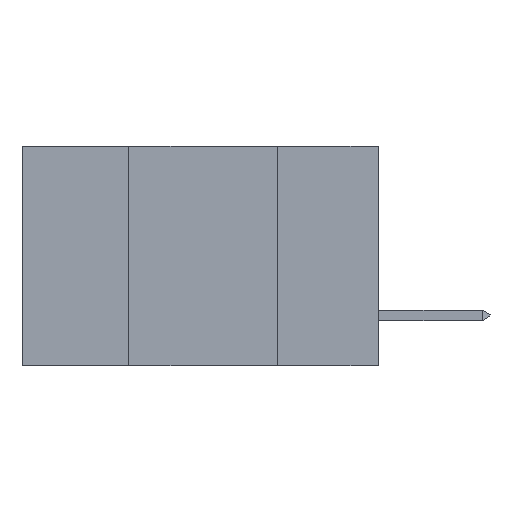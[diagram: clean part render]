
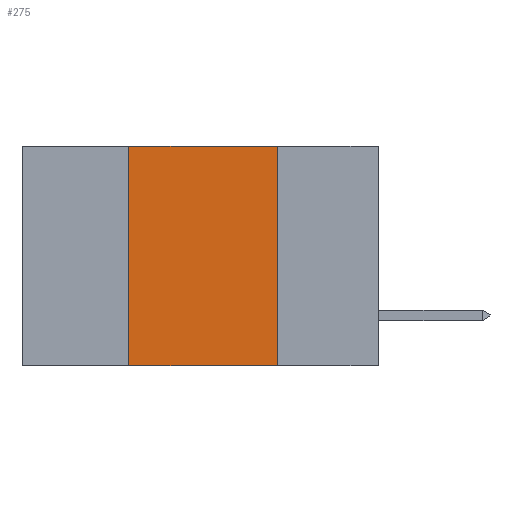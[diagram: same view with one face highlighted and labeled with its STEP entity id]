
A CAD part, left-side view. The second image highlights one B-rep face of the part: STEP entity #275.
In plain terms, the highlighted planar face has unit normal (-1, 0, 0).
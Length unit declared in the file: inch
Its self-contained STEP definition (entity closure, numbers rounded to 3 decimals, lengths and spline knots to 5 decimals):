
#275 = ADVANCED_FACE ( 'NONE', ( #8260 ), #2193, .F. ) ;
#759 = DIRECTION ( 'NONE',  ( 0., 0., 1. ) ) ;
#766 = EDGE_CURVE ( 'NONE', #15417, #3319, #3799, .T. ) ;
#1206 = CARTESIAN_POINT ( 'NONE',  ( 0., 0.17, -0.37 ) ) ;
#1298 = ORIENTED_EDGE ( 'NONE', *, *, #3155, .F. ) ;
#1468 = CARTESIAN_POINT ( 'NONE',  ( 0., 0.6, -0.37 ) ) ;
#1653 = VECTOR ( 'NONE', #8609, 39.37008 ) ;
#2193 = PLANE ( 'NONE',  #11209 ) ;
#2322 = CARTESIAN_POINT ( 'NONE',  ( 0., 0.17, -0.37 ) ) ;
#2664 = CARTESIAN_POINT ( 'NONE',  ( 0., 0.42, 0. ) ) ;
#3048 = CARTESIAN_POINT ( 'NONE',  ( 0., 0.17, 0. ) ) ;
#3155 = EDGE_CURVE ( 'NONE', #15417, #5871, #3295, .T. ) ;
#3295 = LINE ( 'NONE', #15176, #4633 ) ;
#3316 = DIRECTION ( 'NONE',  ( 0., 0., -1. ) ) ;
#3319 = VERTEX_POINT ( 'NONE', #1206 ) ;
#3799 = LINE ( 'NONE', #1468, #1653 ) ;
#4366 = DIRECTION ( 'NONE',  ( 0., -1., 0. ) ) ;
#4633 = VECTOR ( 'NONE', #759, 39.37008 ) ;
#4879 = VERTEX_POINT ( 'NONE', #3048 ) ;
#5771 = ORIENTED_EDGE ( 'NONE', *, *, #14552, .F. ) ;
#5833 = EDGE_CURVE ( 'NONE', #4879, #3319, #10586, .T. ) ;
#5871 = VERTEX_POINT ( 'NONE', #2664 ) ;
#7837 = VECTOR ( 'NONE', #3316, 39.37008 ) ;
#8143 = ORIENTED_EDGE ( 'NONE', *, *, #5833, .F. ) ;
#8184 = CARTESIAN_POINT ( 'NONE',  ( 0., 0.6, 0. ) ) ;
#8260 = FACE_OUTER_BOUND ( 'NONE', #11651, .T. ) ;
#8609 = DIRECTION ( 'NONE',  ( 0., -1., 0. ) ) ;
#10586 = LINE ( 'NONE', #2322, #7837 ) ;
#10707 = CARTESIAN_POINT ( 'NONE',  ( 0., 0.42, -0.37 ) ) ;
#11209 = AXIS2_PLACEMENT_3D ( 'NONE', #8184, #13171, #13088 ) ;
#11651 = EDGE_LOOP ( 'NONE', ( #8143, #5771, #1298, #14617 ) ) ;
#11789 = VECTOR ( 'NONE', #4366, 39.37008 ) ;
#13088 = DIRECTION ( 'NONE',  ( 0., 0., -1. ) ) ;
#13171 = DIRECTION ( 'NONE',  ( 1., 0., 0. ) ) ;
#14043 = LINE ( 'NONE', #15148, #11789 ) ;
#14552 = EDGE_CURVE ( 'NONE', #5871, #4879, #14043, .T. ) ;
#14617 = ORIENTED_EDGE ( 'NONE', *, *, #766, .T. ) ;
#15148 = CARTESIAN_POINT ( 'NONE',  ( 0., 0.6, 0. ) ) ;
#15176 = CARTESIAN_POINT ( 'NONE',  ( 0., 0.42, -0.37 ) ) ;
#15417 = VERTEX_POINT ( 'NONE', #10707 ) ;
